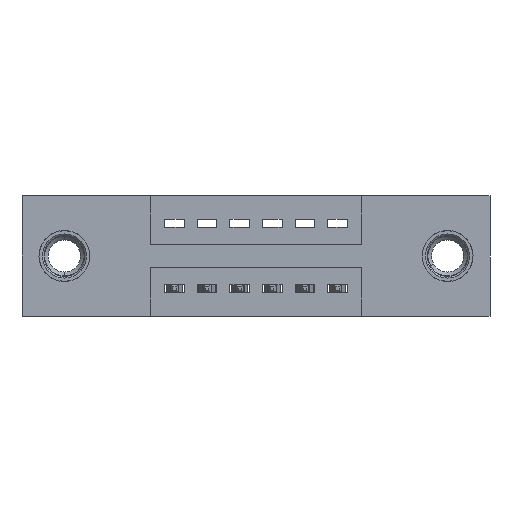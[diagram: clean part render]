
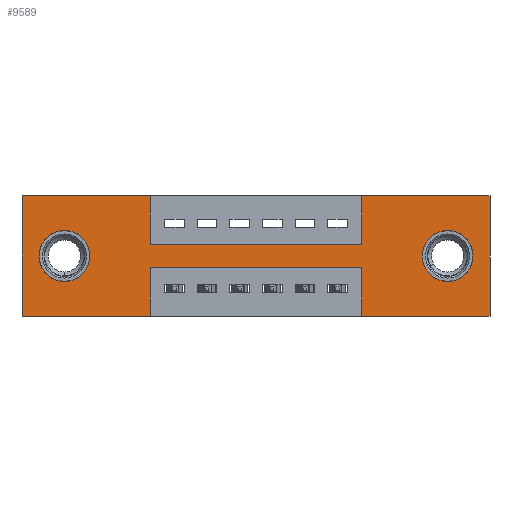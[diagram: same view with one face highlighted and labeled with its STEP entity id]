
A CAD part, front view. The second image highlights one B-rep face of the part: STEP entity #9589.
In plain terms, the highlighted planar face has unit normal (0, -1, 0).
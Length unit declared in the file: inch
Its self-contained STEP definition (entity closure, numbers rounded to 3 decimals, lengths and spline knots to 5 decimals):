
#14 = DIRECTION ( 'NONE',  ( 0., 0., 1. ) ) ;
#60 = DIRECTION ( 'NONE',  ( 0., 0., -1. ) ) ;
#94 = VECTOR ( 'NONE', #2644, 39.37008 ) ;
#236 = LINE ( 'NONE', #5559, #8411 ) ;
#245 = VECTOR ( 'NONE', #60, 39.37008 ) ;
#351 = CARTESIAN_POINT ( 'NONE',  ( 0.3925, 0., -0.15 ) ) ;
#373 = LINE ( 'NONE', #9948, #245 ) ;
#381 = VERTEX_POINT ( 'NONE', #6246 ) ;
#403 = ORIENTED_EDGE ( 'NONE', *, *, #8734, .T. ) ;
#452 = FACE_BOUND ( 'NONE', #8845, .T. ) ;
#529 = CARTESIAN_POINT ( 'NONE',  ( 0., 0., -0.37 ) ) ;
#659 = DIRECTION ( 'NONE',  ( 0., 0., -1. ) ) ;
#745 = VECTOR ( 'NONE', #2131, 39.37008 ) ;
#760 = LINE ( 'NONE', #529, #3449 ) ;
#785 = EDGE_CURVE ( 'NONE', #9801, #9591, #2618, .T. ) ;
#996 = CARTESIAN_POINT ( 'NONE',  ( 0.3925, 0., -0.37 ) ) ;
#1046 = CARTESIAN_POINT ( 'NONE',  ( 0.13, 0., -0.185 ) ) ;
#1112 = DIRECTION ( 'NONE',  ( 0., 1., 0. ) ) ;
#1136 = DIRECTION ( 'NONE',  ( 0., 0., -1. ) ) ;
#1153 = DIRECTION ( 'NONE',  ( -1., 0., 0. ) ) ;
#1163 = VERTEX_POINT ( 'NONE', #996 ) ;
#1171 = VECTOR ( 'NONE', #1136, 39.37008 ) ;
#1338 = DIRECTION ( 'NONE',  ( -1., 0., 0. ) ) ;
#1408 = DIRECTION ( 'NONE',  ( 0., -1., 0. ) ) ;
#1437 = VERTEX_POINT ( 'NONE', #9720 ) ;
#1596 = VERTEX_POINT ( 'NONE', #8250 ) ;
#1623 = ORIENTED_EDGE ( 'NONE', *, *, #4447, .F. ) ;
#1754 = VERTEX_POINT ( 'NONE', #5315 ) ;
#1808 = ORIENTED_EDGE ( 'NONE', *, *, #9762, .F. ) ;
#1870 = CARTESIAN_POINT ( 'NONE',  ( 0.3925, 0., 0. ) ) ;
#1896 = CARTESIAN_POINT ( 'NONE',  ( 0., 0., 0. ) ) ;
#1950 = CARTESIAN_POINT ( 'NONE',  ( 0., 0., -0.37 ) ) ;
#2131 = DIRECTION ( 'NONE',  ( 1., 0., 0. ) ) ;
#2191 = CARTESIAN_POINT ( 'NONE',  ( 1.435, 0., -0.37 ) ) ;
#2234 = CARTESIAN_POINT ( 'NONE',  ( 1.305, 0., -0.185 ) ) ;
#2247 = LINE ( 'NONE', #1896, #94 ) ;
#2314 = CIRCLE ( 'NONE', #7678, 0.078 ) ;
#2329 = CARTESIAN_POINT ( 'NONE',  ( 1.435, 0., 0. ) ) ;
#2348 = VECTOR ( 'NONE', #10385, 39.37008 ) ;
#2379 = EDGE_LOOP ( 'NONE', ( #9845, #2616, #1623, #7200, #7262, #5384, #4248, #5625, #3226, #9803, #1808, #7353 ) ) ;
#2420 = CARTESIAN_POINT ( 'NONE',  ( 0., 0., 0. ) ) ;
#2553 = CARTESIAN_POINT ( 'NONE',  ( 1.0425, 0., 0. ) ) ;
#2555 = EDGE_CURVE ( 'NONE', #1754, #4975, #2314, .T. ) ;
#2616 = ORIENTED_EDGE ( 'NONE', *, *, #8949, .F. ) ;
#2618 = LINE ( 'NONE', #2329, #5318 ) ;
#2621 = FACE_OUTER_BOUND ( 'NONE', #2379, .T. ) ;
#2644 = DIRECTION ( 'NONE',  ( 0., 0., 1. ) ) ;
#2756 = VECTOR ( 'NONE', #1153, 39.37008 ) ;
#2782 = CARTESIAN_POINT ( 'NONE',  ( 1.435, 0., 0. ) ) ;
#2919 = LINE ( 'NONE', #8673, #745 ) ;
#3046 = VERTEX_POINT ( 'NONE', #1870 ) ;
#3226 = ORIENTED_EDGE ( 'NONE', *, *, #7456, .F. ) ;
#3449 = VECTOR ( 'NONE', #1338, 39.37008 ) ;
#3624 = EDGE_CURVE ( 'NONE', #5372, #3046, #3968, .T. ) ;
#3660 = CARTESIAN_POINT ( 'NONE',  ( 0.3925, 0., -0.22 ) ) ;
#3738 = LINE ( 'NONE', #4477, #1171 ) ;
#3757 = LINE ( 'NONE', #4551, #2348 ) ;
#3868 = EDGE_CURVE ( 'NONE', #1163, #8921, #760, .T. ) ;
#3968 = LINE ( 'NONE', #7593, #5896 ) ;
#3995 = DIRECTION ( 'NONE',  ( 0., 1., 0. ) ) ;
#4181 = DIRECTION ( 'NONE',  ( 0., 0., -1. ) ) ;
#4248 = ORIENTED_EDGE ( 'NONE', *, *, #9939, .F. ) ;
#4306 = CARTESIAN_POINT ( 'NONE',  ( 1.0425, 0., -0.22 ) ) ;
#4318 = EDGE_LOOP ( 'NONE', ( #4718, #403 ) ) ;
#4394 = DIRECTION ( 'NONE',  ( 1., 0., 0. ) ) ;
#4447 = EDGE_CURVE ( 'NONE', #7505, #9729, #3757, .T. ) ;
#4477 = CARTESIAN_POINT ( 'NONE',  ( 0.3925, 0., -0.37 ) ) ;
#4530 = LINE ( 'NONE', #2553, #7508 ) ;
#4551 = CARTESIAN_POINT ( 'NONE',  ( 1.0425, 0., -0.37 ) ) ;
#4718 = ORIENTED_EDGE ( 'NONE', *, *, #2555, .T. ) ;
#4769 = AXIS2_PLACEMENT_3D ( 'NONE', #1950, #1408, #659 ) ;
#4814 = DIRECTION ( 'NONE',  ( 0., 0., -1. ) ) ;
#4815 = AXIS2_PLACEMENT_3D ( 'NONE', #2234, #3995, #4814 ) ;
#4816 = CARTESIAN_POINT ( 'NONE',  ( 0.13, 0., -0.185 ) ) ;
#4850 = DIRECTION ( 'NONE',  ( 0., 0., 1. ) ) ;
#4863 = CIRCLE ( 'NONE', #4815, 0.078 ) ;
#4928 = CARTESIAN_POINT ( 'NONE',  ( 0.13, 0., -0.263 ) ) ;
#4975 = VERTEX_POINT ( 'NONE', #4928 ) ;
#5048 = CARTESIAN_POINT ( 'NONE',  ( 1.0425, 0., -0.37 ) ) ;
#5201 = PLANE ( 'NONE',  #4769 ) ;
#5242 = CARTESIAN_POINT ( 'NONE',  ( 0., 0., -0.37 ) ) ;
#5294 = VERTEX_POINT ( 'NONE', #351 ) ;
#5310 = DIRECTION ( 'NONE',  ( 0., 0., -1. ) ) ;
#5315 = CARTESIAN_POINT ( 'NONE',  ( 0.13, 0., -0.107 ) ) ;
#5318 = VECTOR ( 'NONE', #4181, 39.37008 ) ;
#5372 = VERTEX_POINT ( 'NONE', #2420 ) ;
#5384 = ORIENTED_EDGE ( 'NONE', *, *, #7589, .F. ) ;
#5536 = EDGE_CURVE ( 'NONE', #1437, #1163, #3738, .T. ) ;
#5559 = CARTESIAN_POINT ( 'NONE',  ( 0., 0., -0.37 ) ) ;
#5625 = ORIENTED_EDGE ( 'NONE', *, *, #8553, .F. ) ;
#5645 = DIRECTION ( 'NONE',  ( 0., 1., 0. ) ) ;
#5706 = FACE_BOUND ( 'NONE', #4318, .T. ) ;
#5819 = ORIENTED_EDGE ( 'NONE', *, *, #6934, .T. ) ;
#5896 = VECTOR ( 'NONE', #9212, 39.37008 ) ;
#6179 = CARTESIAN_POINT ( 'NONE',  ( 1.305, 0., -0.185 ) ) ;
#6235 = CIRCLE ( 'NONE', #10319, 0.078 ) ;
#6246 = CARTESIAN_POINT ( 'NONE',  ( 1.305, 0., -0.107 ) ) ;
#6484 = LINE ( 'NONE', #3660, #2756 ) ;
#6538 = VERTEX_POINT ( 'NONE', #6645 ) ;
#6645 = CARTESIAN_POINT ( 'NONE',  ( 1.305, 0., -0.263 ) ) ;
#6828 = DIRECTION ( 'NONE',  ( 0., 0., 1. ) ) ;
#6934 = EDGE_CURVE ( 'NONE', #381, #6538, #4863, .T. ) ;
#7200 = ORIENTED_EDGE ( 'NONE', *, *, #8294, .F. ) ;
#7250 = DIRECTION ( 'NONE',  ( -1., 0., 0. ) ) ;
#7262 = ORIENTED_EDGE ( 'NONE', *, *, #785, .F. ) ;
#7353 = ORIENTED_EDGE ( 'NONE', *, *, #3868, .F. ) ;
#7456 = EDGE_CURVE ( 'NONE', #3046, #5294, #373, .T. ) ;
#7505 = VERTEX_POINT ( 'NONE', #5048 ) ;
#7508 = VECTOR ( 'NONE', #14, 39.37008 ) ;
#7589 = EDGE_CURVE ( 'NONE', #8972, #9801, #2919, .T. ) ;
#7593 = CARTESIAN_POINT ( 'NONE',  ( 0., 0., 0. ) ) ;
#7678 = AXIS2_PLACEMENT_3D ( 'NONE', #4816, #5645, #4850 ) ;
#7832 = DIRECTION ( 'NONE',  ( 0., 1., 0. ) ) ;
#8042 = LINE ( 'NONE', #10075, #8653 ) ;
#8250 = CARTESIAN_POINT ( 'NONE',  ( 1.0425, 0., -0.15 ) ) ;
#8294 = EDGE_CURVE ( 'NONE', #9591, #7505, #236, .T. ) ;
#8411 = VECTOR ( 'NONE', #7250, 39.37008 ) ;
#8553 = EDGE_CURVE ( 'NONE', #5294, #1596, #8042, .T. ) ;
#8653 = VECTOR ( 'NONE', #4394, 39.37008 ) ;
#8673 = CARTESIAN_POINT ( 'NONE',  ( 0., 0., 0. ) ) ;
#8734 = EDGE_CURVE ( 'NONE', #4975, #1754, #10574, .T. ) ;
#8828 = EDGE_CURVE ( 'NONE', #6538, #381, #6235, .T. ) ;
#8845 = EDGE_LOOP ( 'NONE', ( #5819, #9236 ) ) ;
#8921 = VERTEX_POINT ( 'NONE', #5242 ) ;
#8949 = EDGE_CURVE ( 'NONE', #9729, #1437, #6484, .T. ) ;
#8972 = VERTEX_POINT ( 'NONE', #10463 ) ;
#9212 = DIRECTION ( 'NONE',  ( 1., 0., 0. ) ) ;
#9214 = AXIS2_PLACEMENT_3D ( 'NONE', #1046, #1112, #6828 ) ;
#9236 = ORIENTED_EDGE ( 'NONE', *, *, #8828, .T. ) ;
#9589 = ADVANCED_FACE ( 'NONE', ( #452, #5706, #2621 ), #5201, .T. ) ;
#9591 = VERTEX_POINT ( 'NONE', #2191 ) ;
#9720 = CARTESIAN_POINT ( 'NONE',  ( 0.3925, 0., -0.22 ) ) ;
#9729 = VERTEX_POINT ( 'NONE', #4306 ) ;
#9762 = EDGE_CURVE ( 'NONE', #8921, #5372, #2247, .T. ) ;
#9801 = VERTEX_POINT ( 'NONE', #2782 ) ;
#9803 = ORIENTED_EDGE ( 'NONE', *, *, #3624, .F. ) ;
#9845 = ORIENTED_EDGE ( 'NONE', *, *, #5536, .F. ) ;
#9939 = EDGE_CURVE ( 'NONE', #1596, #8972, #4530, .T. ) ;
#9948 = CARTESIAN_POINT ( 'NONE',  ( 0.3925, 0., 0. ) ) ;
#10075 = CARTESIAN_POINT ( 'NONE',  ( 0.3925, 0., -0.15 ) ) ;
#10319 = AXIS2_PLACEMENT_3D ( 'NONE', #6179, #7832, #5310 ) ;
#10385 = DIRECTION ( 'NONE',  ( 0., 0., 1. ) ) ;
#10463 = CARTESIAN_POINT ( 'NONE',  ( 1.0425, 0., 0. ) ) ;
#10574 = CIRCLE ( 'NONE', #9214, 0.078 ) ;
